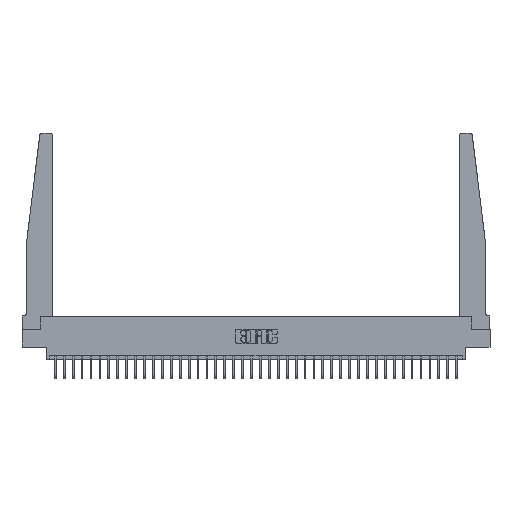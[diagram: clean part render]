
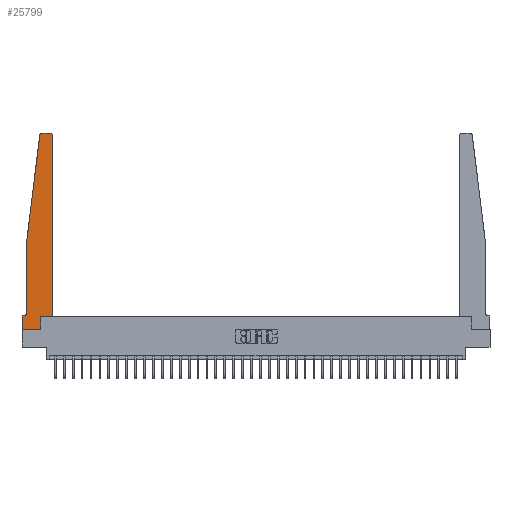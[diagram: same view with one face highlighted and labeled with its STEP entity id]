
A CAD part, top view. The second image highlights one B-rep face of the part: STEP entity #25799.
In plain terms, the highlighted planar face has unit normal (0, 0, 1).
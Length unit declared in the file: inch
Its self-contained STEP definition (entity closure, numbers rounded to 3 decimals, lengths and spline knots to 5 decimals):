
#469 = DIRECTION ( 'NONE',  ( 0., -1., 0. ) ) ;
#758 = VERTEX_POINT ( 'NONE', #25604 ) ;
#769 = ORIENTED_EDGE ( 'NONE', *, *, #13543, .T. ) ;
#852 = DIRECTION ( 'NONE',  ( 0., 0., 1. ) ) ;
#1569 = VERTEX_POINT ( 'NONE', #9312 ) ;
#1607 = VECTOR ( 'NONE', #14208, 39.37008 ) ;
#2078 = VERTEX_POINT ( 'NONE', #29337 ) ;
#2241 = ORIENTED_EDGE ( 'NONE', *, *, #22922, .T. ) ;
#2619 = VECTOR ( 'NONE', #30328, 39.37008 ) ;
#2705 = LINE ( 'NONE', #10474, #7962 ) ;
#2724 = VERTEX_POINT ( 'NONE', #29520 ) ;
#2912 = AXIS2_PLACEMENT_3D ( 'NONE', #14042, #31684, #16609 ) ;
#5425 = CARTESIAN_POINT ( 'NONE',  ( 0.015, 0.1875, 0.37 ) ) ;
#5488 = ORIENTED_EDGE ( 'NONE', *, *, #14370, .T. ) ;
#6204 = DIRECTION ( 'NONE',  ( -0.122, -0.992, 0. ) ) ;
#6301 = ORIENTED_EDGE ( 'NONE', *, *, #9946, .T. ) ;
#6399 = DIRECTION ( 'NONE',  ( 0., 0., 1. ) ) ;
#6953 = EDGE_CURVE ( 'NONE', #2724, #1569, #26522, .T. ) ;
#7170 = VERTEX_POINT ( 'NONE', #28013 ) ;
#7886 = CARTESIAN_POINT ( 'NONE',  ( 0.395, 2.72, 0.37 ) ) ;
#7962 = VECTOR ( 'NONE', #23261, 39.37008 ) ;
#8505 = LINE ( 'NONE', #14096, #1607 ) ;
#8903 = VECTOR ( 'NONE', #469, 39.37008 ) ;
#9312 = CARTESIAN_POINT ( 'NONE',  ( 0.065, 0.2375, 0.37 ) ) ;
#9565 = VERTEX_POINT ( 'NONE', #17310 ) ;
#9946 = EDGE_CURVE ( 'NONE', #1569, #29906, #31788, .T. ) ;
#10061 = ORIENTED_EDGE ( 'NONE', *, *, #28826, .T. ) ;
#10066 = CARTESIAN_POINT ( 'NONE',  ( 0.25, 2.75, 0.37 ) ) ;
#10076 = ORIENTED_EDGE ( 'NONE', *, *, #26843, .T. ) ;
#10141 = VECTOR ( 'NONE', #6204, 39.37008 ) ;
#10460 = DIRECTION ( 'NONE',  ( 1., 0., 0. ) ) ;
#10474 = CARTESIAN_POINT ( 'NONE',  ( 0.425, 0.18, 0.37 ) ) ;
#11052 = CARTESIAN_POINT ( 'NONE',  ( 0.395, 2.75, 0.37 ) ) ;
#11124 = ORIENTED_EDGE ( 'NONE', *, *, #22686, .T. ) ;
#11429 = CARTESIAN_POINT ( 'NONE',  ( 0.24675, 2.72367, 0.37 ) ) ;
#11597 = EDGE_LOOP ( 'NONE', ( #5488, #769, #10061, #12559, #6301, #13738, #11124, #15371, #2241, #27240, #16391, #10076 ) ) ;
#12559 = ORIENTED_EDGE ( 'NONE', *, *, #6953, .T. ) ;
#12766 = EDGE_CURVE ( 'NONE', #758, #9565, #30985, .T. ) ;
#13009 = CARTESIAN_POINT ( 'NONE',  ( 0., 0.1875, 0.37 ) ) ;
#13543 = EDGE_CURVE ( 'NONE', #7170, #16535, #21513, .T. ) ;
#13738 = ORIENTED_EDGE ( 'NONE', *, *, #20076, .T. ) ;
#13988 = AXIS2_PLACEMENT_3D ( 'NONE', #7886, #25664, #10460 ) ;
#13995 = PLANE ( 'NONE',  #27763 ) ;
#14042 = CARTESIAN_POINT ( 'NONE',  ( 0.015, 0.2375, 0.37 ) ) ;
#14096 = CARTESIAN_POINT ( 'NONE',  ( 0.2605, 0.18, 0.37 ) ) ;
#14208 = DIRECTION ( 'NONE',  ( 0., 1., 0. ) ) ;
#14370 = EDGE_CURVE ( 'NONE', #18822, #7170, #17090, .T. ) ;
#15371 = ORIENTED_EDGE ( 'NONE', *, *, #12766, .T. ) ;
#16276 = CARTESIAN_POINT ( 'NONE',  ( 0.27653, 2.72, 0.37 ) ) ;
#16391 = ORIENTED_EDGE ( 'NONE', *, *, #25045, .T. ) ;
#16535 = VERTEX_POINT ( 'NONE', #11429 ) ;
#16609 = DIRECTION ( 'NONE',  ( -1., 0., 0. ) ) ;
#16890 = DIRECTION ( 'NONE',  ( 0., -1., 0. ) ) ;
#17090 = LINE ( 'NONE', #10066, #2619 ) ;
#17310 = CARTESIAN_POINT ( 'NONE',  ( 0.2605, 0., 0.37 ) ) ;
#18232 = CARTESIAN_POINT ( 'NONE',  ( 0.065, 0.1875, 0.37 ) ) ;
#18440 = CARTESIAN_POINT ( 'NONE',  ( 0., 0., 0.37 ) ) ;
#18757 = EDGE_CURVE ( 'NONE', #2078, #32778, #19984, .T. ) ;
#18822 = VERTEX_POINT ( 'NONE', #11052 ) ;
#18834 = DIRECTION ( 'NONE',  ( 1., 0., 0. ) ) ;
#18932 = CARTESIAN_POINT ( 'NONE',  ( 0.065, 1.25, 0.37 ) ) ;
#19984 = LINE ( 'NONE', #23410, #26681 ) ;
#20076 = EDGE_CURVE ( 'NONE', #29906, #29233, #27765, .T. ) ;
#20287 = FACE_OUTER_BOUND ( 'NONE', #11597, .T. ) ;
#21074 = CIRCLE ( 'NONE', #13988, 0.03 ) ;
#21513 = CIRCLE ( 'NONE', #29622, 0.03 ) ;
#21677 = CARTESIAN_POINT ( 'NONE',  ( 0., 0.1875, 0.37 ) ) ;
#22686 = EDGE_CURVE ( 'NONE', #29233, #758, #23251, .T. ) ;
#22893 = LINE ( 'NONE', #18932, #10141 ) ;
#22922 = EDGE_CURVE ( 'NONE', #9565, #2078, #8505, .T. ) ;
#23251 = LINE ( 'NONE', #23439, #8903 ) ;
#23261 = DIRECTION ( 'NONE',  ( 0., 1., 0. ) ) ;
#23410 = CARTESIAN_POINT ( 'NONE',  ( 0.425, 0.18, 0.37 ) ) ;
#23439 = CARTESIAN_POINT ( 'NONE',  ( 0., 0., 0.37 ) ) ;
#24194 = DIRECTION ( 'NONE',  ( 1., 0., 0. ) ) ;
#24310 = VECTOR ( 'NONE', #26046, 39.37008 ) ;
#25045 = EDGE_CURVE ( 'NONE', #32778, #31924, #2705, .T. ) ;
#25381 = VECTOR ( 'NONE', #25855, 39.37008 ) ;
#25604 = CARTESIAN_POINT ( 'NONE',  ( 0., 0., 0.37 ) ) ;
#25664 = DIRECTION ( 'NONE',  ( 0., 0., 1. ) ) ;
#25799 = ADVANCED_FACE ( 'NONE', ( #20287 ), #13995, .T. ) ;
#25855 = DIRECTION ( 'NONE',  ( -1., 0., 0. ) ) ;
#25931 = DIRECTION ( 'NONE',  ( 1., 0., 0. ) ) ;
#26046 = DIRECTION ( 'NONE',  ( 1., 0., 0. ) ) ;
#26522 = LINE ( 'NONE', #29442, #32381 ) ;
#26681 = VECTOR ( 'NONE', #25931, 39.37008 ) ;
#26843 = EDGE_CURVE ( 'NONE', #31924, #18822, #21074, .T. ) ;
#27240 = ORIENTED_EDGE ( 'NONE', *, *, #18757, .T. ) ;
#27763 = AXIS2_PLACEMENT_3D ( 'NONE', #21677, #6399, #24194 ) ;
#27765 = LINE ( 'NONE', #18232, #25381 ) ;
#28013 = CARTESIAN_POINT ( 'NONE',  ( 0.27653, 2.75, 0.37 ) ) ;
#28826 = EDGE_CURVE ( 'NONE', #16535, #2724, #22893, .T. ) ;
#29233 = VERTEX_POINT ( 'NONE', #13009 ) ;
#29337 = CARTESIAN_POINT ( 'NONE',  ( 0.2605, 0.18, 0.37 ) ) ;
#29442 = CARTESIAN_POINT ( 'NONE',  ( 0.065, 1.25, 0.37 ) ) ;
#29520 = CARTESIAN_POINT ( 'NONE',  ( 0.065, 1.25, 0.37 ) ) ;
#29622 = AXIS2_PLACEMENT_3D ( 'NONE', #16276, #852, #18834 ) ;
#29906 = VERTEX_POINT ( 'NONE', #5425 ) ;
#30328 = DIRECTION ( 'NONE',  ( -1., 0., 0. ) ) ;
#30985 = LINE ( 'NONE', #18440, #24310 ) ;
#31192 = CARTESIAN_POINT ( 'NONE',  ( 0.425, 0.18, 0.37 ) ) ;
#31684 = DIRECTION ( 'NONE',  ( 0., 0., -1. ) ) ;
#31785 = CARTESIAN_POINT ( 'NONE',  ( 0.425, 2.72, 0.37 ) ) ;
#31788 = CIRCLE ( 'NONE', #2912, 0.05 ) ;
#31924 = VERTEX_POINT ( 'NONE', #31785 ) ;
#32381 = VECTOR ( 'NONE', #16890, 39.37008 ) ;
#32778 = VERTEX_POINT ( 'NONE', #31192 ) ;
